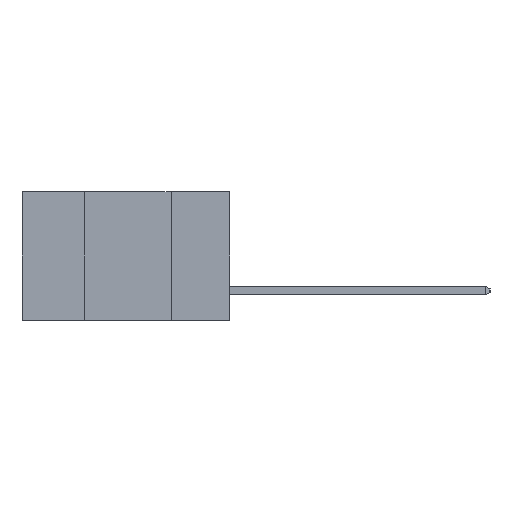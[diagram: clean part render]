
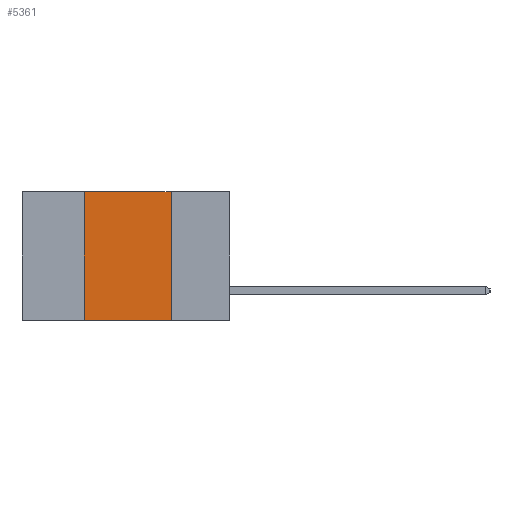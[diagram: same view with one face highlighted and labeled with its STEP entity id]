
A CAD part, left-side view. The second image highlights one B-rep face of the part: STEP entity #5361.
In plain terms, the highlighted planar face has unit normal (-1, 0, 0).
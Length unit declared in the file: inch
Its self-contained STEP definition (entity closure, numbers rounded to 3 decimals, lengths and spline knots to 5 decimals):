
#141 = CARTESIAN_POINT ( 'NONE',  ( 0., 0.17, 0. ) ) ;
#310 = DIRECTION ( 'NONE',  ( 0., 0., -1. ) ) ;
#312 = DIRECTION ( 'NONE',  ( 1., 0., 0. ) ) ;
#594 = EDGE_LOOP ( 'NONE', ( #3949, #3716, #1359, #1271 ) ) ;
#1271 = ORIENTED_EDGE ( 'NONE', *, *, #6136, .T. ) ;
#1359 = ORIENTED_EDGE ( 'NONE', *, *, #3130, .F. ) ;
#2165 = LINE ( 'NONE', #3315, #8135 ) ;
#2699 = EDGE_CURVE ( 'NONE', #7254, #4072, #4982, .T. ) ;
#2754 = VECTOR ( 'NONE', #5200, 39.37008 ) ;
#3130 = EDGE_CURVE ( 'NONE', #3148, #7254, #5778, .T. ) ;
#3148 = VERTEX_POINT ( 'NONE', #10343 ) ;
#3187 = AXIS2_PLACEMENT_3D ( 'NONE', #6467, #312, #310 ) ;
#3315 = CARTESIAN_POINT ( 'NONE',  ( 0., 0.6, -0.37 ) ) ;
#3404 = DIRECTION ( 'NONE',  ( 0., -1., 0. ) ) ;
#3669 = CARTESIAN_POINT ( 'NONE',  ( 0., 0.42, 0. ) ) ;
#3716 = ORIENTED_EDGE ( 'NONE', *, *, #2699, .F. ) ;
#3741 = CARTESIAN_POINT ( 'NONE',  ( 0., 0.17, 0. ) ) ;
#3949 = ORIENTED_EDGE ( 'NONE', *, *, #7111, .F. ) ;
#4072 = VERTEX_POINT ( 'NONE', #141 ) ;
#4526 = LINE ( 'NONE', #3741, #6705 ) ;
#4765 = VERTEX_POINT ( 'NONE', #9980 ) ;
#4982 = LINE ( 'NONE', #6473, #2754 ) ;
#5200 = DIRECTION ( 'NONE',  ( 0., -1., 0. ) ) ;
#5361 = ADVANCED_FACE ( 'NONE', ( #9452 ), #8651, .F. ) ;
#5519 = VECTOR ( 'NONE', #10030, 39.37008 ) ;
#5778 = LINE ( 'NONE', #10053, #5519 ) ;
#6136 = EDGE_CURVE ( 'NONE', #3148, #4765, #2165, .T. ) ;
#6467 = CARTESIAN_POINT ( 'NONE',  ( 0., 0.6, 0. ) ) ;
#6473 = CARTESIAN_POINT ( 'NONE',  ( 0., 0.6, 0. ) ) ;
#6705 = VECTOR ( 'NONE', #7946, 39.37008 ) ;
#7111 = EDGE_CURVE ( 'NONE', #4072, #4765, #4526, .T. ) ;
#7254 = VERTEX_POINT ( 'NONE', #3669 ) ;
#7946 = DIRECTION ( 'NONE',  ( 0., 0., -1. ) ) ;
#8135 = VECTOR ( 'NONE', #3404, 39.37008 ) ;
#8651 = PLANE ( 'NONE',  #3187 ) ;
#9452 = FACE_OUTER_BOUND ( 'NONE', #594, .T. ) ;
#9980 = CARTESIAN_POINT ( 'NONE',  ( 0., 0.17, -0.37 ) ) ;
#10030 = DIRECTION ( 'NONE',  ( 0., 0., 1. ) ) ;
#10053 = CARTESIAN_POINT ( 'NONE',  ( 0., 0.42, 0. ) ) ;
#10343 = CARTESIAN_POINT ( 'NONE',  ( 0., 0.42, -0.37 ) ) ;
